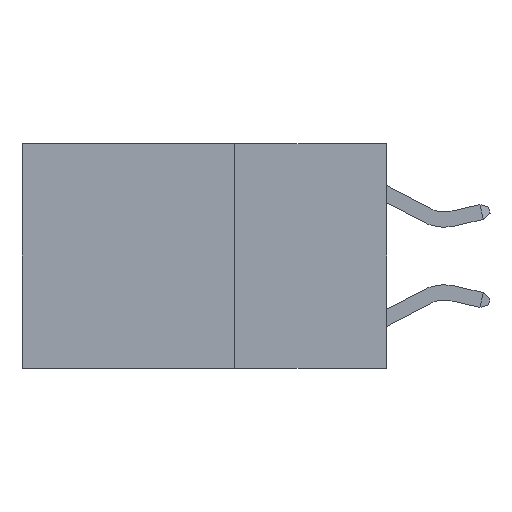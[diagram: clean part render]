
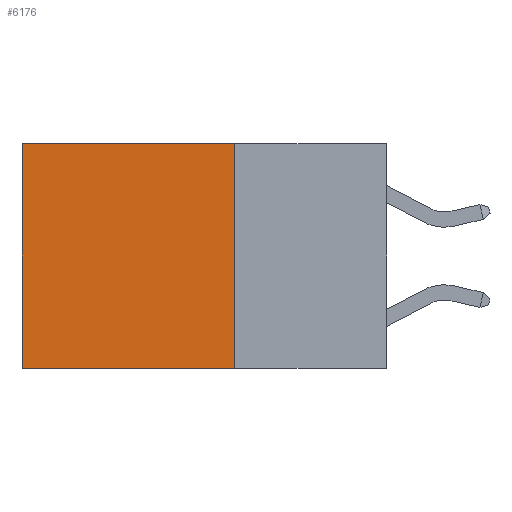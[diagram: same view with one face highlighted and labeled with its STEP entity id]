
A CAD part, left-side view. The second image highlights one B-rep face of the part: STEP entity #6176.
In plain terms, the highlighted planar face has unit normal (-1, 0, 0).
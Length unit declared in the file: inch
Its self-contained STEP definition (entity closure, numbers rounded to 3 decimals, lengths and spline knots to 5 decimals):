
#253 = EDGE_CURVE ( 'NONE', #19116, #1015, #2977, .T. ) ;
#394 = VECTOR ( 'NONE', #9849, 39.37008 ) ;
#605 = VERTEX_POINT ( 'NONE', #6576 ) ;
#1015 = VERTEX_POINT ( 'NONE', #14628 ) ;
#1521 = EDGE_LOOP ( 'NONE', ( #1533, #5962, #7014, #18195 ) ) ;
#1533 = ORIENTED_EDGE ( 'NONE', *, *, #1601, .T. ) ;
#1593 = CARTESIAN_POINT ( 'NONE',  ( 0.2625, 0.25, 0. ) ) ;
#1601 = EDGE_CURVE ( 'NONE', #605, #1015, #12976, .T. ) ;
#2076 = EDGE_CURVE ( 'NONE', #8264, #19116, #12491, .T. ) ;
#2977 = LINE ( 'NONE', #16163, #6543 ) ;
#3237 = DIRECTION ( 'NONE',  ( 0., 0., -1. ) ) ;
#3471 = CARTESIAN_POINT ( 'NONE',  ( 0.2625, 0.25, 0. ) ) ;
#5962 = ORIENTED_EDGE ( 'NONE', *, *, #253, .F. ) ;
#6176 = ADVANCED_FACE ( 'NONE', ( #6803 ), #6235, .F. ) ;
#6235 = PLANE ( 'NONE',  #15271 ) ;
#6543 = VECTOR ( 'NONE', #13159, 39.37008 ) ;
#6576 = CARTESIAN_POINT ( 'NONE',  ( 0.2625, 0.6, 0. ) ) ;
#6803 = FACE_OUTER_BOUND ( 'NONE', #1521, .T. ) ;
#7014 = ORIENTED_EDGE ( 'NONE', *, *, #2076, .F. ) ;
#8264 = VERTEX_POINT ( 'NONE', #15670 ) ;
#9849 = DIRECTION ( 'NONE',  ( 0., 0., -1. ) ) ;
#10301 = DIRECTION ( 'NONE',  ( 0., 0., -1. ) ) ;
#11972 = LINE ( 'NONE', #3471, #18946 ) ;
#12140 = DIRECTION ( 'NONE',  ( 1., 0., 0. ) ) ;
#12491 = LINE ( 'NONE', #18696, #394 ) ;
#12525 = EDGE_CURVE ( 'NONE', #8264, #605, #11972, .T. ) ;
#12976 = LINE ( 'NONE', #17674, #16481 ) ;
#13159 = DIRECTION ( 'NONE',  ( 0., 1., 0. ) ) ;
#14628 = CARTESIAN_POINT ( 'NONE',  ( 0.2625, 0.6, -0.37 ) ) ;
#15271 = AXIS2_PLACEMENT_3D ( 'NONE', #1593, #12140, #3237 ) ;
#15368 = DIRECTION ( 'NONE',  ( 0., 1., 0. ) ) ;
#15670 = CARTESIAN_POINT ( 'NONE',  ( 0.2625, 0.25, 0. ) ) ;
#16163 = CARTESIAN_POINT ( 'NONE',  ( 0.2625, 0.25, -0.37 ) ) ;
#16481 = VECTOR ( 'NONE', #10301, 39.37008 ) ;
#17098 = CARTESIAN_POINT ( 'NONE',  ( 0.2625, 0.25, -0.37 ) ) ;
#17674 = CARTESIAN_POINT ( 'NONE',  ( 0.2625, 0.6, 0. ) ) ;
#18195 = ORIENTED_EDGE ( 'NONE', *, *, #12525, .T. ) ;
#18696 = CARTESIAN_POINT ( 'NONE',  ( 0.2625, 0.25, 0. ) ) ;
#18946 = VECTOR ( 'NONE', #15368, 39.37008 ) ;
#19116 = VERTEX_POINT ( 'NONE', #17098 ) ;
